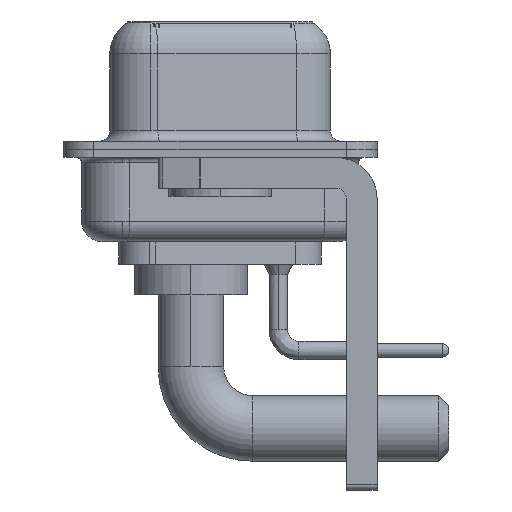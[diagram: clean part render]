
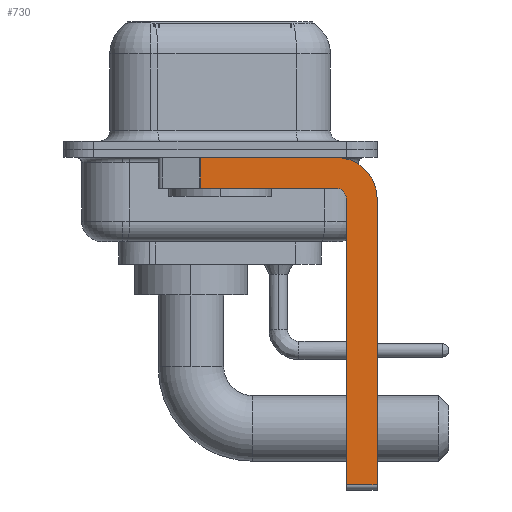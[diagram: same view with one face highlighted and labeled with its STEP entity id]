
A CAD part, left-side view. The second image highlights one B-rep face of the part: STEP entity #730.
In plain terms, the highlighted planar face has unit normal (-1, 0, 0).
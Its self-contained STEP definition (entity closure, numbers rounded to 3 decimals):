
#550 = CARTESIAN_POINT ( 'NONE',  ( -2.9, -5.65, -2.4 ) ) ;
#730 = ADVANCED_FACE ( 'NONE', ( #5764 ), #17658, .F. ) ;
#873 = VERTEX_POINT ( 'NONE', #13091 ) ;
#1619 = ORIENTED_EDGE ( 'NONE', *, *, #5948, .F. ) ;
#1706 = DIRECTION ( 'NONE',  ( 1., 0., 0. ) ) ;
#2037 = ORIENTED_EDGE ( 'NONE', *, *, #9777, .F. ) ;
#2224 = AXIS2_PLACEMENT_3D ( 'NONE', #17075, #13743, #15628 ) ;
#2435 = DIRECTION ( 'NONE',  ( 0., 0., 1. ) ) ;
#2693 = VERTEX_POINT ( 'NONE', #20660 ) ;
#3100 = EDGE_CURVE ( 'NONE', #873, #19990, #20236, .T. ) ;
#3358 = ORIENTED_EDGE ( 'NONE', *, *, #3388, .F. ) ;
#3388 = EDGE_CURVE ( 'NONE', #2693, #6826, #16202, .T. ) ;
#3422 = EDGE_LOOP ( 'NONE', ( #21499, #3700, #3358, #1619, #16431, #10257, #20957, #2037 ) ) ;
#3700 = ORIENTED_EDGE ( 'NONE', *, *, #15537, .T. ) ;
#3843 = CARTESIAN_POINT ( 'NONE',  ( -2.9, -5.65, -16.35 ) ) ;
#4298 = VERTEX_POINT ( 'NONE', #10654 ) ;
#4325 = EDGE_CURVE ( 'NONE', #9793, #8168, #14088, .T. ) ;
#4806 = AXIS2_PLACEMENT_3D ( 'NONE', #550, #21111, #17440 ) ;
#4979 = VECTOR ( 'NONE', #2435, 1000. ) ;
#5215 = DIRECTION ( 'NONE',  ( 0., 0., -1. ) ) ;
#5254 = CARTESIAN_POINT ( 'NONE',  ( -2.9, -5.65, -2.4 ) ) ;
#5764 = FACE_OUTER_BOUND ( 'NONE', #3422, .T. ) ;
#5948 = EDGE_CURVE ( 'NONE', #8168, #2693, #15323, .T. ) ;
#6671 = VECTOR ( 'NONE', #16586, 1000. ) ;
#6826 = VERTEX_POINT ( 'NONE', #11879 ) ;
#7031 = CARTESIAN_POINT ( 'NONE',  ( -2.9, -6.15, -16.35 ) ) ;
#8168 = VERTEX_POINT ( 'NONE', #15006 ) ;
#8957 = DIRECTION ( 'NONE',  ( 0., -1., 0. ) ) ;
#8984 = CARTESIAN_POINT ( 'NONE',  ( -2.9, -6.15, -16.6 ) ) ;
#9777 = EDGE_CURVE ( 'NONE', #12461, #873, #21048, .T. ) ;
#9793 = VERTEX_POINT ( 'NONE', #7031 ) ;
#9824 = VECTOR ( 'NONE', #17533, 1000. ) ;
#10257 = ORIENTED_EDGE ( 'NONE', *, *, #13364, .T. ) ;
#10539 = CARTESIAN_POINT ( 'NONE',  ( -2.9, -7.65, -2.4 ) ) ;
#10626 = VECTOR ( 'NONE', #19032, 1000. ) ;
#10654 = CARTESIAN_POINT ( 'NONE',  ( -2.9, 0.978, -0.4 ) ) ;
#10769 = CARTESIAN_POINT ( 'NONE',  ( -2.9, -5.65, -1.9 ) ) ;
#11456 = AXIS2_PLACEMENT_3D ( 'NONE', #5254, #1706, #15470 ) ;
#11879 = CARTESIAN_POINT ( 'NONE',  ( -2.9, 0.978, -1.9 ) ) ;
#12439 = CARTESIAN_POINT ( 'NONE',  ( -2.9, -5.65, -0.4 ) ) ;
#12461 = VERTEX_POINT ( 'NONE', #12439 ) ;
#12556 = CARTESIAN_POINT ( 'NONE',  ( -2.9, -7.65, -16.35 ) ) ;
#13091 = CARTESIAN_POINT ( 'NONE',  ( -2.9, -7.65, -2.4 ) ) ;
#13364 = EDGE_CURVE ( 'NONE', #9793, #19990, #19074, .T. ) ;
#13743 = DIRECTION ( 'NONE',  ( -1., 0., 0. ) ) ;
#14088 = LINE ( 'NONE', #8984, #4979 ) ;
#15006 = CARTESIAN_POINT ( 'NONE',  ( -2.9, -6.15, -2.4 ) ) ;
#15141 = LINE ( 'NONE', #21936, #6671 ) ;
#15323 = CIRCLE ( 'NONE', #2224, 0.5 ) ;
#15470 = DIRECTION ( 'NONE',  ( 0., 0., -1. ) ) ;
#15537 = EDGE_CURVE ( 'NONE', #4298, #6826, #15141, .T. ) ;
#15628 = DIRECTION ( 'NONE',  ( 0., 0., 1. ) ) ;
#16164 = VECTOR ( 'NONE', #8957, 1000. ) ;
#16202 = LINE ( 'NONE', #10769, #9824 ) ;
#16431 = ORIENTED_EDGE ( 'NONE', *, *, #4325, .F. ) ;
#16560 = VECTOR ( 'NONE', #5215, 1000. ) ;
#16586 = DIRECTION ( 'NONE',  ( 0., 0., -1. ) ) ;
#17075 = CARTESIAN_POINT ( 'NONE',  ( -2.9, -5.65, -2.4 ) ) ;
#17440 = DIRECTION ( 'NONE',  ( 0., 0., -1. ) ) ;
#17533 = DIRECTION ( 'NONE',  ( 0., 1., 0. ) ) ;
#17658 = PLANE ( 'NONE',  #4806 ) ;
#18924 = LINE ( 'NONE', #20698, #10626 ) ;
#19032 = DIRECTION ( 'NONE',  ( 0., -1., 0. ) ) ;
#19074 = LINE ( 'NONE', #3843, #16164 ) ;
#19990 = VERTEX_POINT ( 'NONE', #12556 ) ;
#20236 = LINE ( 'NONE', #10539, #16560 ) ;
#20660 = CARTESIAN_POINT ( 'NONE',  ( -2.9, -5.65, -1.9 ) ) ;
#20698 = CARTESIAN_POINT ( 'NONE',  ( -2.9, 3., -0.4 ) ) ;
#20841 = EDGE_CURVE ( 'NONE', #4298, #12461, #18924, .T. ) ;
#20957 = ORIENTED_EDGE ( 'NONE', *, *, #3100, .F. ) ;
#21048 = CIRCLE ( 'NONE', #11456, 2. ) ;
#21111 = DIRECTION ( 'NONE',  ( 1., 0., 0. ) ) ;
#21499 = ORIENTED_EDGE ( 'NONE', *, *, #20841, .F. ) ;
#21936 = CARTESIAN_POINT ( 'NONE',  ( -2.9, 0.978, -1.9 ) ) ;
